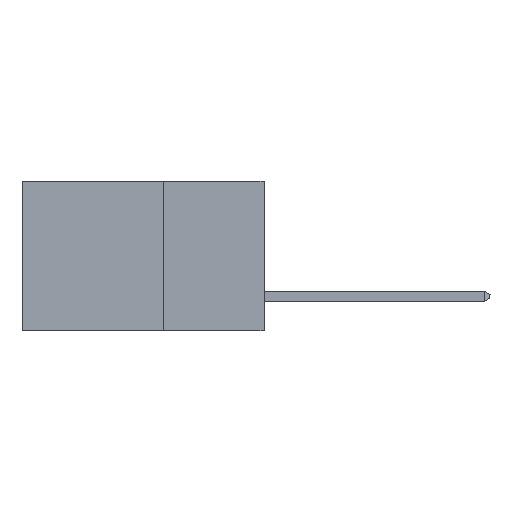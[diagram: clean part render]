
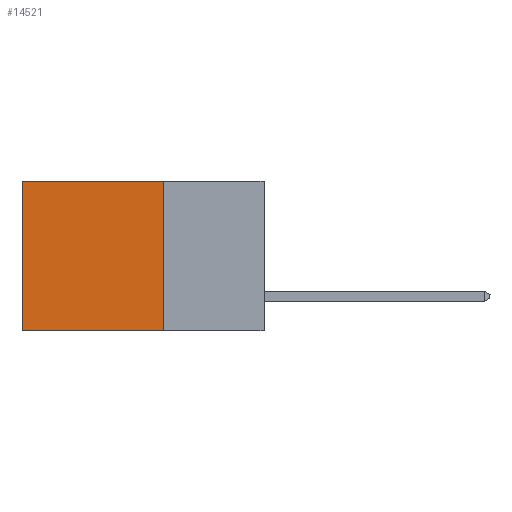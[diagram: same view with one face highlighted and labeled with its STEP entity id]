
A CAD part, left-side view. The second image highlights one B-rep face of the part: STEP entity #14521.
In plain terms, the highlighted planar face has unit normal (-1, 0, 0).
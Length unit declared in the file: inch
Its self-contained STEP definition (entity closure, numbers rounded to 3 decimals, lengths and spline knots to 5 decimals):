
#188 = VECTOR ( 'NONE', #6883, 39.37008 ) ;
#236 = EDGE_CURVE ( 'NONE', #1098, #15575, #3615, .T. ) ;
#1098 = VERTEX_POINT ( 'NONE', #4863 ) ;
#1417 = EDGE_CURVE ( 'NONE', #1098, #11492, #8575, .T. ) ;
#1464 = CARTESIAN_POINT ( 'NONE',  ( 0.2615, 0.25, 0. ) ) ;
#1607 = VECTOR ( 'NONE', #17730, 39.37008 ) ;
#2932 = CARTESIAN_POINT ( 'NONE',  ( 0.2615, 0.6, -0.37 ) ) ;
#3600 = LINE ( 'NONE', #12207, #1607 ) ;
#3615 = LINE ( 'NONE', #4910, #6349 ) ;
#3937 = FACE_OUTER_BOUND ( 'NONE', #9797, .T. ) ;
#4201 = DIRECTION ( 'NONE',  ( 0., 0., -1. ) ) ;
#4863 = CARTESIAN_POINT ( 'NONE',  ( 0.2615, 0.25, 0. ) ) ;
#4910 = CARTESIAN_POINT ( 'NONE',  ( 0.2615, 0.25, -0.37 ) ) ;
#5585 = DIRECTION ( 'NONE',  ( 1., 0., 0. ) ) ;
#6349 = VECTOR ( 'NONE', #17115, 39.37008 ) ;
#6883 = DIRECTION ( 'NONE',  ( 0., 0., -1. ) ) ;
#8419 = VERTEX_POINT ( 'NONE', #14360 ) ;
#8575 = LINE ( 'NONE', #1464, #14187 ) ;
#9495 = AXIS2_PLACEMENT_3D ( 'NONE', #16686, #5585, #4201 ) ;
#9797 = EDGE_LOOP ( 'NONE', ( #10789, #15380, #16642, #14834 ) ) ;
#10789 = ORIENTED_EDGE ( 'NONE', *, *, #17165, .T. ) ;
#11094 = LINE ( 'NONE', #2932, #188 ) ;
#11492 = VERTEX_POINT ( 'NONE', #17629 ) ;
#11543 = CARTESIAN_POINT ( 'NONE',  ( 0.2615, 0.25, -0.37 ) ) ;
#12207 = CARTESIAN_POINT ( 'NONE',  ( 0.2615, 0.25, -0.37 ) ) ;
#14112 = DIRECTION ( 'NONE',  ( 0., 1., 0. ) ) ;
#14187 = VECTOR ( 'NONE', #14112, 39.37008 ) ;
#14360 = CARTESIAN_POINT ( 'NONE',  ( 0.2615, 0.6, -0.37 ) ) ;
#14521 = ADVANCED_FACE ( 'NONE', ( #3937 ), #17870, .F. ) ;
#14834 = ORIENTED_EDGE ( 'NONE', *, *, #1417, .T. ) ;
#15336 = EDGE_CURVE ( 'NONE', #15575, #8419, #3600, .T. ) ;
#15380 = ORIENTED_EDGE ( 'NONE', *, *, #15336, .F. ) ;
#15575 = VERTEX_POINT ( 'NONE', #11543 ) ;
#16642 = ORIENTED_EDGE ( 'NONE', *, *, #236, .F. ) ;
#16686 = CARTESIAN_POINT ( 'NONE',  ( 0.2615, 0.25, -0.37 ) ) ;
#17115 = DIRECTION ( 'NONE',  ( 0., 0., -1. ) ) ;
#17165 = EDGE_CURVE ( 'NONE', #11492, #8419, #11094, .T. ) ;
#17629 = CARTESIAN_POINT ( 'NONE',  ( 0.2615, 0.6, 0. ) ) ;
#17730 = DIRECTION ( 'NONE',  ( 0., 1., 0. ) ) ;
#17870 = PLANE ( 'NONE',  #9495 ) ;
